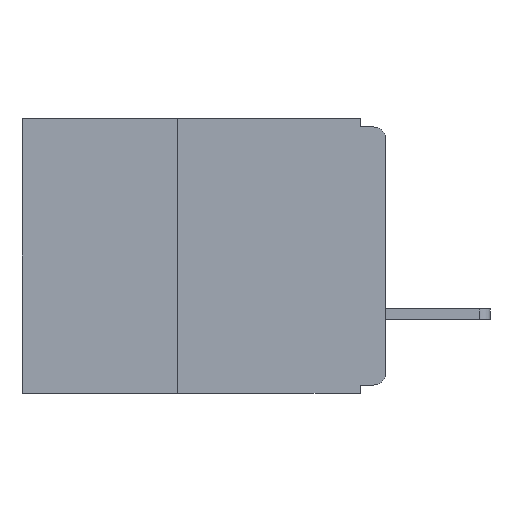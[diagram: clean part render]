
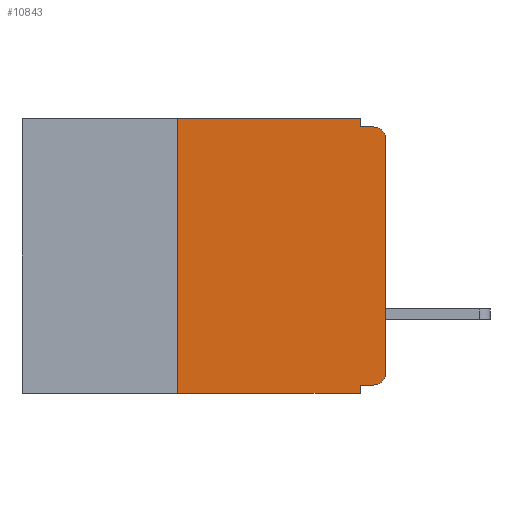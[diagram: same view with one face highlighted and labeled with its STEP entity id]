
A CAD part, left-side view. The second image highlights one B-rep face of the part: STEP entity #10843.
In plain terms, the highlighted planar face has unit normal (-1, 0, 0).
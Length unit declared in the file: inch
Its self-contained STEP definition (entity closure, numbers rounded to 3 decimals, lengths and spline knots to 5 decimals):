
#257 = DIRECTION ( 'NONE',  ( 0., -1., 0. ) ) ;
#515 = CARTESIAN_POINT ( 'NONE',  ( 0., 0., -0.025 ) ) ;
#587 = CARTESIAN_POINT ( 'NONE',  ( 0., 0.437, -0.33 ) ) ;
#1393 = AXIS2_PLACEMENT_3D ( 'NONE', #2007, #23524, #9312 ) ;
#1486 = EDGE_CURVE ( 'NONE', #12124, #22514, #15110, .T. ) ;
#1679 = VERTEX_POINT ( 'NONE', #25528 ) ;
#1707 = EDGE_CURVE ( 'NONE', #12378, #29429, #14706, .T. ) ;
#1709 = VERTEX_POINT ( 'NONE', #24974 ) ;
#2007 = CARTESIAN_POINT ( 'NONE',  ( 0., 0.437, 0. ) ) ;
#2326 = CARTESIAN_POINT ( 'NONE',  ( 0., 0., -0.01 ) ) ;
#2448 = EDGE_CURVE ( 'NONE', #1709, #14376, #24954, .T. ) ;
#2680 = EDGE_CURVE ( 'NONE', #1679, #12378, #12750, .T. ) ;
#2785 = ORIENTED_EDGE ( 'NONE', *, *, #21250, .T. ) ;
#3474 = VERTEX_POINT ( 'NONE', #8969 ) ;
#3495 = CARTESIAN_POINT ( 'NONE',  ( 0., 0.437, 0. ) ) ;
#5006 = VECTOR ( 'NONE', #19133, 39.37008 ) ;
#5362 = EDGE_CURVE ( 'NONE', #12124, #30593, #24057, .T. ) ;
#5389 = EDGE_CURVE ( 'NONE', #14376, #10627, #22591, .T. ) ;
#6995 = DIRECTION ( 'NONE',  ( 0., 0., -1. ) ) ;
#7031 = DIRECTION ( 'NONE',  ( -1., 0., 0. ) ) ;
#7070 = CARTESIAN_POINT ( 'NONE',  ( 0., 0.015, -0.305 ) ) ;
#8028 = CARTESIAN_POINT ( 'NONE',  ( 0., 0.031, -0.33 ) ) ;
#8819 = CARTESIAN_POINT ( 'NONE',  ( 0., 0., -0.32 ) ) ;
#8969 = CARTESIAN_POINT ( 'NONE',  ( 0., 0.031, -0.32 ) ) ;
#9054 = ORIENTED_EDGE ( 'NONE', *, *, #12283, .F. ) ;
#9312 = DIRECTION ( 'NONE',  ( 0., 0., -1. ) ) ;
#9320 = ORIENTED_EDGE ( 'NONE', *, *, #14827, .F. ) ;
#9342 = ORIENTED_EDGE ( 'NONE', *, *, #1486, .F. ) ;
#10315 = LINE ( 'NONE', #3495, #22200 ) ;
#10409 = CARTESIAN_POINT ( 'NONE',  ( 0., 0.25, -0.33 ) ) ;
#10627 = VERTEX_POINT ( 'NONE', #27449 ) ;
#10843 = ADVANCED_FACE ( 'NONE', ( #14401 ), #21172, .F. ) ;
#12124 = VERTEX_POINT ( 'NONE', #10409 ) ;
#12283 = EDGE_CURVE ( 'NONE', #1679, #3474, #29324, .T. ) ;
#12378 = VERTEX_POINT ( 'NONE', #13995 ) ;
#12425 = CARTESIAN_POINT ( 'NONE',  ( 0., 0.015, -0.025 ) ) ;
#12561 = CARTESIAN_POINT ( 'NONE',  ( 0., 0.031, 0. ) ) ;
#12750 = CIRCLE ( 'NONE', #20294, 0.015 ) ;
#13259 = DIRECTION ( 'NONE',  ( 0., 0., -1. ) ) ;
#13962 = VECTOR ( 'NONE', #25013, 39.37008 ) ;
#13995 = CARTESIAN_POINT ( 'NONE',  ( 0., 0., -0.305 ) ) ;
#14376 = VERTEX_POINT ( 'NONE', #16409 ) ;
#14401 = FACE_OUTER_BOUND ( 'NONE', #24051, .T. ) ;
#14706 = LINE ( 'NONE', #25257, #13962 ) ;
#14827 = EDGE_CURVE ( 'NONE', #22514, #1709, #10315, .T. ) ;
#14839 = DIRECTION ( 'NONE',  ( 0., 0., -1. ) ) ;
#15110 = LINE ( 'NONE', #29122, #26855 ) ;
#16125 = ORIENTED_EDGE ( 'NONE', *, *, #1707, .T. ) ;
#16409 = CARTESIAN_POINT ( 'NONE',  ( 0., 0.031, -0.01 ) ) ;
#16509 = ORIENTED_EDGE ( 'NONE', *, *, #2680, .T. ) ;
#16586 = ORIENTED_EDGE ( 'NONE', *, *, #22014, .F. ) ;
#17117 = VECTOR ( 'NONE', #257, 39.37008 ) ;
#17618 = DIRECTION ( 'NONE',  ( 0., 0., -1. ) ) ;
#18702 = VECTOR ( 'NONE', #13259, 39.37008 ) ;
#18848 = VECTOR ( 'NONE', #17618, 39.37008 ) ;
#19133 = DIRECTION ( 'NONE',  ( 0., -1., 0. ) ) ;
#19513 = AXIS2_PLACEMENT_3D ( 'NONE', #12425, #28838, #14839 ) ;
#19581 = LINE ( 'NONE', #8028, #18848 ) ;
#20294 = AXIS2_PLACEMENT_3D ( 'NONE', #7070, #7031, #6995 ) ;
#21172 = PLANE ( 'NONE',  #1393 ) ;
#21250 = EDGE_CURVE ( 'NONE', #29429, #10627, #22516, .T. ) ;
#21337 = CARTESIAN_POINT ( 'NONE',  ( 0., 0.25, 0. ) ) ;
#22014 = EDGE_CURVE ( 'NONE', #3474, #30593, #19581, .T. ) ;
#22200 = VECTOR ( 'NONE', #22709, 39.37008 ) ;
#22514 = VERTEX_POINT ( 'NONE', #21337 ) ;
#22516 = CIRCLE ( 'NONE', #19513, 0.015 ) ;
#22591 = LINE ( 'NONE', #2326, #5006 ) ;
#22709 = DIRECTION ( 'NONE',  ( 0., -1., 0. ) ) ;
#23524 = DIRECTION ( 'NONE',  ( 1., 0., 0. ) ) ;
#24051 = EDGE_LOOP ( 'NONE', ( #16125, #2785, #26984, #26468, #9320, #9342, #30581, #16586, #9054, #16509 ) ) ;
#24057 = LINE ( 'NONE', #587, #17117 ) ;
#24412 = CARTESIAN_POINT ( 'NONE',  ( 0., 0.031, -0.33 ) ) ;
#24954 = LINE ( 'NONE', #12561, #18702 ) ;
#24974 = CARTESIAN_POINT ( 'NONE',  ( 0., 0.031, 0. ) ) ;
#25013 = DIRECTION ( 'NONE',  ( 0., 0., 1. ) ) ;
#25257 = CARTESIAN_POINT ( 'NONE',  ( 0., 0., 0. ) ) ;
#25528 = CARTESIAN_POINT ( 'NONE',  ( 0., 0.015, -0.32 ) ) ;
#26468 = ORIENTED_EDGE ( 'NONE', *, *, #2448, .F. ) ;
#26855 = VECTOR ( 'NONE', #29287, 39.37008 ) ;
#26984 = ORIENTED_EDGE ( 'NONE', *, *, #5389, .F. ) ;
#27449 = CARTESIAN_POINT ( 'NONE',  ( 0., 0.015, -0.01 ) ) ;
#28590 = VECTOR ( 'NONE', #30052, 39.37008 ) ;
#28838 = DIRECTION ( 'NONE',  ( -1., 0., 0. ) ) ;
#29122 = CARTESIAN_POINT ( 'NONE',  ( 0., 0.25, -0.33 ) ) ;
#29287 = DIRECTION ( 'NONE',  ( 0., 0., 1. ) ) ;
#29324 = LINE ( 'NONE', #8819, #28590 ) ;
#29429 = VERTEX_POINT ( 'NONE', #515 ) ;
#30052 = DIRECTION ( 'NONE',  ( 0., 1., 0. ) ) ;
#30581 = ORIENTED_EDGE ( 'NONE', *, *, #5362, .T. ) ;
#30593 = VERTEX_POINT ( 'NONE', #24412 ) ;
